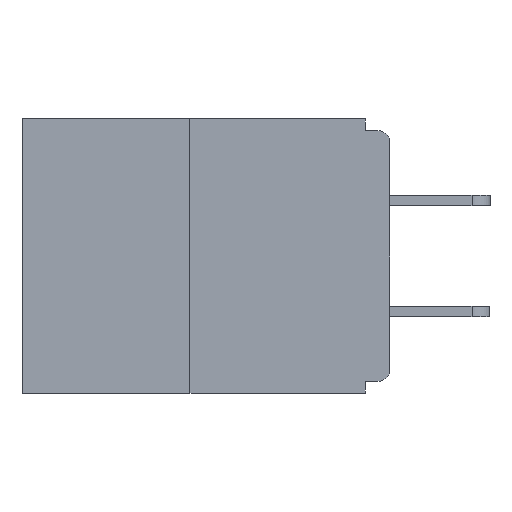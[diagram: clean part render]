
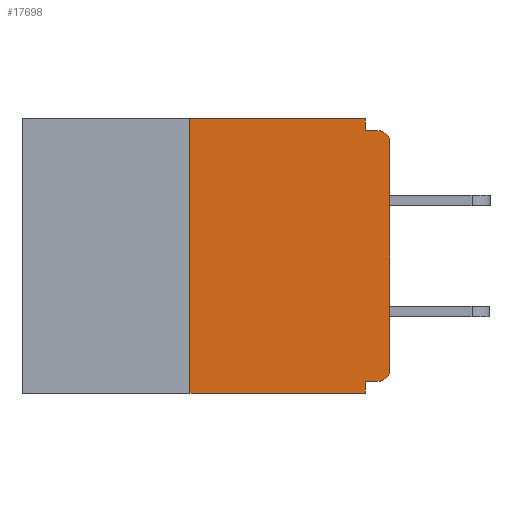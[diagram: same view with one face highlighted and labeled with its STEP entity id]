
A CAD part, left-side view. The second image highlights one B-rep face of the part: STEP entity #17698.
In plain terms, the highlighted planar face has unit normal (-1, 0, 0).
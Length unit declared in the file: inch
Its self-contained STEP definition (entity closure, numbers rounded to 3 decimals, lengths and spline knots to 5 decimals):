
#186 = LINE ( 'NONE', #15825, #3575 ) ;
#403 = CARTESIAN_POINT ( 'NONE',  ( 0., 0.46, -0.343 ) ) ;
#412 = EDGE_CURVE ( 'NONE', #3304, #9269, #5471, .T. ) ;
#664 = DIRECTION ( 'NONE',  ( 0., 1., 0. ) ) ;
#1070 = CARTESIAN_POINT ( 'NONE',  ( 0., 0., -0.313 ) ) ;
#1175 = LINE ( 'NONE', #10772, #16061 ) ;
#1440 = DIRECTION ( 'NONE',  ( 0., 0., -1. ) ) ;
#1574 = EDGE_CURVE ( 'NONE', #11728, #10680, #6547, .T. ) ;
#1615 = PLANE ( 'NONE',  #8696 ) ;
#1731 = CARTESIAN_POINT ( 'NONE',  ( 0., 0.46, 0. ) ) ;
#1751 = EDGE_CURVE ( 'NONE', #14954, #12524, #14264, .T. ) ;
#2078 = AXIS2_PLACEMENT_3D ( 'NONE', #15028, #6200, #7767 ) ;
#2448 = DIRECTION ( 'NONE',  ( 0., 0., 1. ) ) ;
#2521 = CARTESIAN_POINT ( 'NONE',  ( 0., 0.46, 0. ) ) ;
#2940 = ORIENTED_EDGE ( 'NONE', *, *, #17513, .T. ) ;
#2948 = DIRECTION ( 'NONE',  ( -1., 0., 0. ) ) ;
#3304 = VERTEX_POINT ( 'NONE', #17904 ) ;
#3343 = CARTESIAN_POINT ( 'NONE',  ( 0., 0.015, -0.328 ) ) ;
#3447 = DIRECTION ( 'NONE',  ( 0., -1., 0. ) ) ;
#3575 = VECTOR ( 'NONE', #5676, 39.37008 ) ;
#3893 = DIRECTION ( 'NONE',  ( 0., -1., 0. ) ) ;
#4085 = CARTESIAN_POINT ( 'NONE',  ( 0., 0.015, -0.015 ) ) ;
#4841 = VERTEX_POINT ( 'NONE', #10486 ) ;
#5052 = ORIENTED_EDGE ( 'NONE', *, *, #5610, .F. ) ;
#5471 = LINE ( 'NONE', #403, #12863 ) ;
#5610 = EDGE_CURVE ( 'NONE', #3304, #14954, #6610, .T. ) ;
#5649 = CARTESIAN_POINT ( 'NONE',  ( 0., 0., -0.03 ) ) ;
#5676 = DIRECTION ( 'NONE',  ( 0., 0., -1. ) ) ;
#5857 = EDGE_CURVE ( 'NONE', #14776, #11728, #12959, .T. ) ;
#5974 = DIRECTION ( 'NONE',  ( 0., 0., -1. ) ) ;
#6127 = VECTOR ( 'NONE', #3893, 39.37008 ) ;
#6200 = DIRECTION ( 'NONE',  ( -1., 0., 0. ) ) ;
#6547 = CIRCLE ( 'NONE', #2078, 0.015 ) ;
#6610 = LINE ( 'NONE', #8192, #14772 ) ;
#7093 = ORIENTED_EDGE ( 'NONE', *, *, #16621, .F. ) ;
#7153 = LINE ( 'NONE', #15623, #8518 ) ;
#7367 = AXIS2_PLACEMENT_3D ( 'NONE', #9806, #2948, #15934 ) ;
#7616 = CARTESIAN_POINT ( 'NONE',  ( 0., 0., 0. ) ) ;
#7754 = CARTESIAN_POINT ( 'NONE',  ( 0., 0.031, -0.015 ) ) ;
#7767 = DIRECTION ( 'NONE',  ( 0., 0., -1. ) ) ;
#8068 = CARTESIAN_POINT ( 'NONE',  ( 0., 0.25, 0. ) ) ;
#8093 = VECTOR ( 'NONE', #664, 39.37008 ) ;
#8192 = CARTESIAN_POINT ( 'NONE',  ( 0., 0.25, 0. ) ) ;
#8518 = VECTOR ( 'NONE', #1440, 39.37008 ) ;
#8696 = AXIS2_PLACEMENT_3D ( 'NONE', #1731, #8852, #5974 ) ;
#8852 = DIRECTION ( 'NONE',  ( 1., 0., 0. ) ) ;
#9269 = VERTEX_POINT ( 'NONE', #13273 ) ;
#9449 = DIRECTION ( 'NONE',  ( 0., -1., 0. ) ) ;
#9806 = CARTESIAN_POINT ( 'NONE',  ( 0., 0.015, -0.313 ) ) ;
#9860 = EDGE_CURVE ( 'NONE', #13137, #10680, #1175, .T. ) ;
#10079 = CARTESIAN_POINT ( 'NONE',  ( 0., 0.031, 0. ) ) ;
#10486 = CARTESIAN_POINT ( 'NONE',  ( 0., 0.031, -0.328 ) ) ;
#10680 = VERTEX_POINT ( 'NONE', #4085 ) ;
#10772 = CARTESIAN_POINT ( 'NONE',  ( 0., 0., -0.015 ) ) ;
#10937 = CARTESIAN_POINT ( 'NONE',  ( 0., 0., -0.328 ) ) ;
#11728 = VERTEX_POINT ( 'NONE', #5649 ) ;
#12025 = ORIENTED_EDGE ( 'NONE', *, *, #1574, .T. ) ;
#12083 = DIRECTION ( 'NONE',  ( 0., 0., 1. ) ) ;
#12490 = VECTOR ( 'NONE', #12083, 39.37008 ) ;
#12524 = VERTEX_POINT ( 'NONE', #10079 ) ;
#12565 = ORIENTED_EDGE ( 'NONE', *, *, #16998, .F. ) ;
#12716 = EDGE_CURVE ( 'NONE', #13769, #4841, #14866, .T. ) ;
#12863 = VECTOR ( 'NONE', #3447, 39.37008 ) ;
#12959 = LINE ( 'NONE', #7616, #12490 ) ;
#13137 = VERTEX_POINT ( 'NONE', #7754 ) ;
#13273 = CARTESIAN_POINT ( 'NONE',  ( 0., 0.031, -0.343 ) ) ;
#13661 = ORIENTED_EDGE ( 'NONE', *, *, #412, .T. ) ;
#13769 = VERTEX_POINT ( 'NONE', #3343 ) ;
#14264 = LINE ( 'NONE', #2521, #6127 ) ;
#14374 = CIRCLE ( 'NONE', #7367, 0.015 ) ;
#14552 = ORIENTED_EDGE ( 'NONE', *, *, #5857, .T. ) ;
#14772 = VECTOR ( 'NONE', #2448, 39.37008 ) ;
#14776 = VERTEX_POINT ( 'NONE', #1070 ) ;
#14866 = LINE ( 'NONE', #10937, #8093 ) ;
#14954 = VERTEX_POINT ( 'NONE', #8068 ) ;
#15028 = CARTESIAN_POINT ( 'NONE',  ( 0., 0.015, -0.03 ) ) ;
#15110 = ORIENTED_EDGE ( 'NONE', *, *, #1751, .F. ) ;
#15623 = CARTESIAN_POINT ( 'NONE',  ( 0., 0.031, -0.343 ) ) ;
#15825 = CARTESIAN_POINT ( 'NONE',  ( 0., 0.031, 0. ) ) ;
#15934 = DIRECTION ( 'NONE',  ( 0., 0., -1. ) ) ;
#16061 = VECTOR ( 'NONE', #9449, 39.37008 ) ;
#16083 = EDGE_LOOP ( 'NONE', ( #15110, #5052, #13661, #7093, #17192, #2940, #14552, #12025, #18482, #12565 ) ) ;
#16621 = EDGE_CURVE ( 'NONE', #4841, #9269, #7153, .T. ) ;
#16998 = EDGE_CURVE ( 'NONE', #12524, #13137, #186, .T. ) ;
#17192 = ORIENTED_EDGE ( 'NONE', *, *, #12716, .F. ) ;
#17513 = EDGE_CURVE ( 'NONE', #13769, #14776, #14374, .T. ) ;
#17698 = ADVANCED_FACE ( 'NONE', ( #18418 ), #1615, .F. ) ;
#17904 = CARTESIAN_POINT ( 'NONE',  ( 0., 0.25, -0.343 ) ) ;
#18418 = FACE_OUTER_BOUND ( 'NONE', #16083, .T. ) ;
#18482 = ORIENTED_EDGE ( 'NONE', *, *, #9860, .F. ) ;
